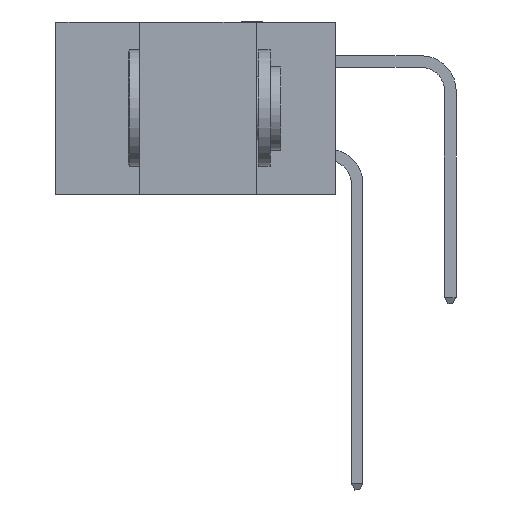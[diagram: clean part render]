
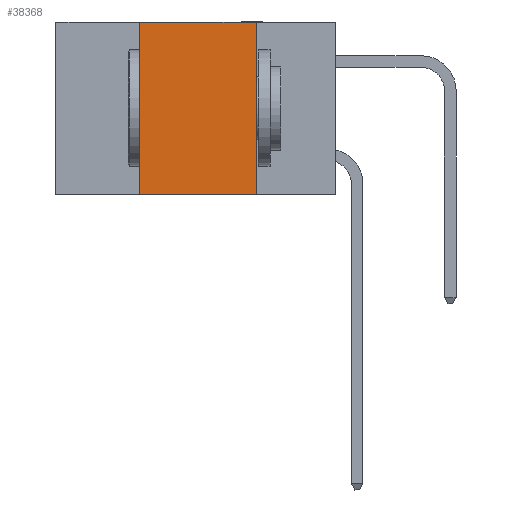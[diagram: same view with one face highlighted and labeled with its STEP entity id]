
A CAD part, left-side view. The second image highlights one B-rep face of the part: STEP entity #38368.
In plain terms, the highlighted planar face has unit normal (-1, 0, 0).
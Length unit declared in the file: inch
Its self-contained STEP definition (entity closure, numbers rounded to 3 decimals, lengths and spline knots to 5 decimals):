
#448 = ORIENTED_EDGE ( 'NONE', *, *, #17848, .T. ) ;
#602 = ORIENTED_EDGE ( 'NONE', *, *, #16258, .F. ) ;
#3018 = LINE ( 'NONE', #33444, #38609 ) ;
#3176 = LINE ( 'NONE', #21438, #22838 ) ;
#5184 = CARTESIAN_POINT ( 'NONE',  ( 0., 0.6, 0. ) ) ;
#8599 = EDGE_CURVE ( 'NONE', #24170, #43549, #3018, .T. ) ;
#9524 = CARTESIAN_POINT ( 'NONE',  ( 0., 0.17, 0. ) ) ;
#11054 = CARTESIAN_POINT ( 'NONE',  ( 0., 0.17, -0.37 ) ) ;
#11174 = VERTEX_POINT ( 'NONE', #11323 ) ;
#11323 = CARTESIAN_POINT ( 'NONE',  ( 0., 0.17, 0. ) ) ;
#12028 = CARTESIAN_POINT ( 'NONE',  ( 0., 0.6, 0. ) ) ;
#12276 = LINE ( 'NONE', #5184, #34621 ) ;
#13528 = FACE_OUTER_BOUND ( 'NONE', #39800, .T. ) ;
#13637 = DIRECTION ( 'NONE',  ( 0., 0., -1. ) ) ;
#14133 = CARTESIAN_POINT ( 'NONE',  ( 0., 0.42, -0.37 ) ) ;
#16258 = EDGE_CURVE ( 'NONE', #11174, #32822, #33757, .T. ) ;
#16667 = CARTESIAN_POINT ( 'NONE',  ( 0., 0.42, 0. ) ) ;
#17520 = ORIENTED_EDGE ( 'NONE', *, *, #8599, .F. ) ;
#17714 = DIRECTION ( 'NONE',  ( 0., -1., 0. ) ) ;
#17848 = EDGE_CURVE ( 'NONE', #24170, #32822, #3176, .T. ) ;
#18301 = PLANE ( 'NONE',  #32866 ) ;
#21024 = VECTOR ( 'NONE', #13637, 39.37008 ) ;
#21438 = CARTESIAN_POINT ( 'NONE',  ( 0., 0.6, -0.37 ) ) ;
#22838 = VECTOR ( 'NONE', #17714, 39.37008 ) ;
#24170 = VERTEX_POINT ( 'NONE', #14133 ) ;
#28322 = DIRECTION ( 'NONE',  ( 0., -1., 0. ) ) ;
#30021 = DIRECTION ( 'NONE',  ( 0., 0., 1. ) ) ;
#32822 = VERTEX_POINT ( 'NONE', #11054 ) ;
#32866 = AXIS2_PLACEMENT_3D ( 'NONE', #12028, #42609, #42007 ) ;
#33444 = CARTESIAN_POINT ( 'NONE',  ( 0., 0.42, 0. ) ) ;
#33753 = EDGE_CURVE ( 'NONE', #43549, #11174, #12276, .T. ) ;
#33757 = LINE ( 'NONE', #9524, #21024 ) ;
#34621 = VECTOR ( 'NONE', #28322, 39.37008 ) ;
#38180 = ORIENTED_EDGE ( 'NONE', *, *, #33753, .F. ) ;
#38368 = ADVANCED_FACE ( 'NONE', ( #13528 ), #18301, .F. ) ;
#38609 = VECTOR ( 'NONE', #30021, 39.37008 ) ;
#39800 = EDGE_LOOP ( 'NONE', ( #602, #38180, #17520, #448 ) ) ;
#42007 = DIRECTION ( 'NONE',  ( 0., 0., -1. ) ) ;
#42609 = DIRECTION ( 'NONE',  ( 1., 0., 0. ) ) ;
#43549 = VERTEX_POINT ( 'NONE', #16667 ) ;
